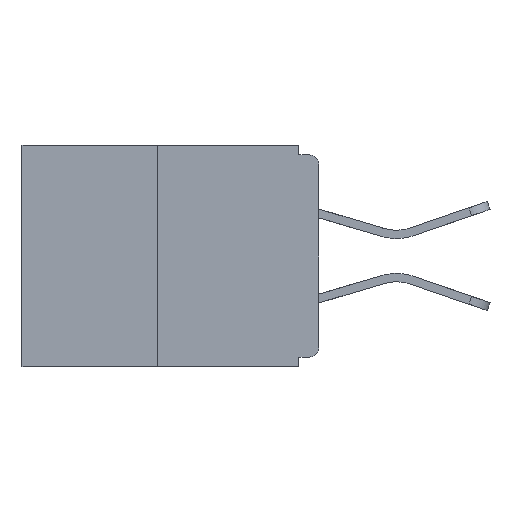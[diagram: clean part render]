
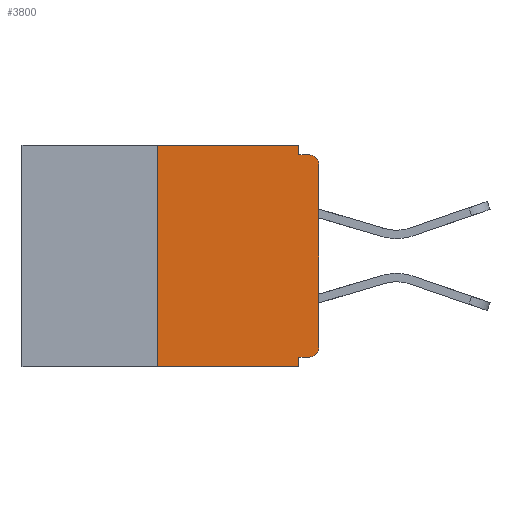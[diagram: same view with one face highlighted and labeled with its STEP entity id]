
A CAD part, left-side view. The second image highlights one B-rep face of the part: STEP entity #3800.
In plain terms, the highlighted planar face has unit normal (-1, 0, 0).
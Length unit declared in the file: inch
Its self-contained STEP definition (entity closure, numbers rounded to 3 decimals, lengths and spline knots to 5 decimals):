
#88 = CIRCLE ( 'NONE', #8862, 0.015 ) ;
#149 = ORIENTED_EDGE ( 'NONE', *, *, #1653, .T. ) ;
#867 = EDGE_CURVE ( 'NONE', #4451, #8676, #1254, .T. ) ;
#878 = CARTESIAN_POINT ( 'NONE',  ( 0., 0.46, 0. ) ) ;
#1254 = LINE ( 'NONE', #12755, #6528 ) ;
#1290 = DIRECTION ( 'NONE',  ( 0., 0., -1. ) ) ;
#1415 = DIRECTION ( 'NONE',  ( 0., 0., -1. ) ) ;
#1560 = LINE ( 'NONE', #2245, #5489 ) ;
#1625 = EDGE_LOOP ( 'NONE', ( #11602, #3511, #5950, #2032, #4675, #11282, #2323, #149, #5816, #4144 ) ) ;
#1653 = EDGE_CURVE ( 'NONE', #7436, #8676, #88, .T. ) ;
#1922 = DIRECTION ( 'NONE',  ( 0., -1., 0. ) ) ;
#2032 = ORIENTED_EDGE ( 'NONE', *, *, #5095, .F. ) ;
#2192 = DIRECTION ( 'NONE',  ( -1., 0., 0. ) ) ;
#2245 = CARTESIAN_POINT ( 'NONE',  ( 0., 0.031, -0.343 ) ) ;
#2323 = ORIENTED_EDGE ( 'NONE', *, *, #8012, .T. ) ;
#2462 = CARTESIAN_POINT ( 'NONE',  ( 0., 0.46, -0.343 ) ) ;
#2469 = VECTOR ( 'NONE', #9025, 39.37008 ) ;
#2713 = EDGE_CURVE ( 'NONE', #13128, #11054, #3749, .T. ) ;
#2714 = AXIS2_PLACEMENT_3D ( 'NONE', #12773, #8467, #8516 ) ;
#2737 = VECTOR ( 'NONE', #9883, 39.37008 ) ;
#2798 = LINE ( 'NONE', #10900, #12561 ) ;
#2830 = LINE ( 'NONE', #5346, #11137 ) ;
#3326 = VERTEX_POINT ( 'NONE', #7584 ) ;
#3511 = ORIENTED_EDGE ( 'NONE', *, *, #9507, .F. ) ;
#3587 = CARTESIAN_POINT ( 'NONE',  ( 0., 0.46, 0. ) ) ;
#3726 = EDGE_CURVE ( 'NONE', #6142, #3326, #10553, .T. ) ;
#3749 = LINE ( 'NONE', #878, #10253 ) ;
#3800 = ADVANCED_FACE ( 'NONE', ( #12673 ), #5524, .F. ) ;
#4144 = ORIENTED_EDGE ( 'NONE', *, *, #11087, .F. ) ;
#4451 = VERTEX_POINT ( 'NONE', #8509 ) ;
#4562 = CARTESIAN_POINT ( 'NONE',  ( 0., 0.25, 0. ) ) ;
#4621 = DIRECTION ( 'NONE',  ( 1., 0., 0. ) ) ;
#4675 = ORIENTED_EDGE ( 'NONE', *, *, #11789, .F. ) ;
#4795 = CARTESIAN_POINT ( 'NONE',  ( 0., 0., -0.328 ) ) ;
#5095 = EDGE_CURVE ( 'NONE', #12539, #3326, #1560, .T. ) ;
#5214 = CARTESIAN_POINT ( 'NONE',  ( 0., 0., -0.03 ) ) ;
#5346 = CARTESIAN_POINT ( 'NONE',  ( 0., 0.25, 0. ) ) ;
#5350 = CARTESIAN_POINT ( 'NONE',  ( 0., 0.015, -0.015 ) ) ;
#5489 = VECTOR ( 'NONE', #7616, 39.37008 ) ;
#5524 = PLANE ( 'NONE',  #6019 ) ;
#5703 = CARTESIAN_POINT ( 'NONE',  ( 0., 0.031, -0.328 ) ) ;
#5816 = ORIENTED_EDGE ( 'NONE', *, *, #867, .F. ) ;
#5950 = ORIENTED_EDGE ( 'NONE', *, *, #3726, .T. ) ;
#6019 = AXIS2_PLACEMENT_3D ( 'NONE', #3587, #4621, #6626 ) ;
#6137 = VECTOR ( 'NONE', #8622, 39.37008 ) ;
#6142 = VERTEX_POINT ( 'NONE', #10043 ) ;
#6291 = CARTESIAN_POINT ( 'NONE',  ( 0., 0.015, -0.328 ) ) ;
#6404 = CARTESIAN_POINT ( 'NONE',  ( 0., 0.015, -0.03 ) ) ;
#6528 = VECTOR ( 'NONE', #9640, 39.37008 ) ;
#6626 = DIRECTION ( 'NONE',  ( 0., 0., -1. ) ) ;
#6685 = CARTESIAN_POINT ( 'NONE',  ( 0., 0., -0.313 ) ) ;
#7436 = VERTEX_POINT ( 'NONE', #5214 ) ;
#7584 = CARTESIAN_POINT ( 'NONE',  ( 0., 0.031, -0.343 ) ) ;
#7616 = DIRECTION ( 'NONE',  ( 0., 0., -1. ) ) ;
#8012 = EDGE_CURVE ( 'NONE', #10164, #7436, #13107, .T. ) ;
#8467 = DIRECTION ( 'NONE',  ( -1., 0., 0. ) ) ;
#8509 = CARTESIAN_POINT ( 'NONE',  ( 0., 0.031, -0.015 ) ) ;
#8516 = DIRECTION ( 'NONE',  ( 0., 0., -1. ) ) ;
#8622 = DIRECTION ( 'NONE',  ( 0., 0., 1. ) ) ;
#8676 = VERTEX_POINT ( 'NONE', #5350 ) ;
#8862 = AXIS2_PLACEMENT_3D ( 'NONE', #6404, #2192, #1290 ) ;
#9025 = DIRECTION ( 'NONE',  ( 0., 1., 0. ) ) ;
#9507 = EDGE_CURVE ( 'NONE', #6142, #13128, #2830, .T. ) ;
#9640 = DIRECTION ( 'NONE',  ( 0., -1., 0. ) ) ;
#9722 = DIRECTION ( 'NONE',  ( 0., 0., 1. ) ) ;
#9755 = CARTESIAN_POINT ( 'NONE',  ( 0., 0., 0. ) ) ;
#9841 = CARTESIAN_POINT ( 'NONE',  ( 0., 0.031, 0. ) ) ;
#9883 = DIRECTION ( 'NONE',  ( 0., -1., 0. ) ) ;
#9905 = VERTEX_POINT ( 'NONE', #6291 ) ;
#10043 = CARTESIAN_POINT ( 'NONE',  ( 0., 0.25, -0.343 ) ) ;
#10164 = VERTEX_POINT ( 'NONE', #6685 ) ;
#10253 = VECTOR ( 'NONE', #1922, 39.37008 ) ;
#10553 = LINE ( 'NONE', #2462, #2737 ) ;
#10900 = CARTESIAN_POINT ( 'NONE',  ( 0., 0.031, 0. ) ) ;
#11054 = VERTEX_POINT ( 'NONE', #9841 ) ;
#11087 = EDGE_CURVE ( 'NONE', #11054, #4451, #2798, .T. ) ;
#11137 = VECTOR ( 'NONE', #9722, 39.37008 ) ;
#11254 = LINE ( 'NONE', #4795, #2469 ) ;
#11282 = ORIENTED_EDGE ( 'NONE', *, *, #12021, .T. ) ;
#11602 = ORIENTED_EDGE ( 'NONE', *, *, #2713, .F. ) ;
#11789 = EDGE_CURVE ( 'NONE', #9905, #12539, #11254, .T. ) ;
#12021 = EDGE_CURVE ( 'NONE', #9905, #10164, #13558, .T. ) ;
#12539 = VERTEX_POINT ( 'NONE', #5703 ) ;
#12561 = VECTOR ( 'NONE', #1415, 39.37008 ) ;
#12673 = FACE_OUTER_BOUND ( 'NONE', #1625, .T. ) ;
#12755 = CARTESIAN_POINT ( 'NONE',  ( 0., 0., -0.015 ) ) ;
#12773 = CARTESIAN_POINT ( 'NONE',  ( 0., 0.015, -0.313 ) ) ;
#13107 = LINE ( 'NONE', #9755, #6137 ) ;
#13128 = VERTEX_POINT ( 'NONE', #4562 ) ;
#13558 = CIRCLE ( 'NONE', #2714, 0.015 ) ;
